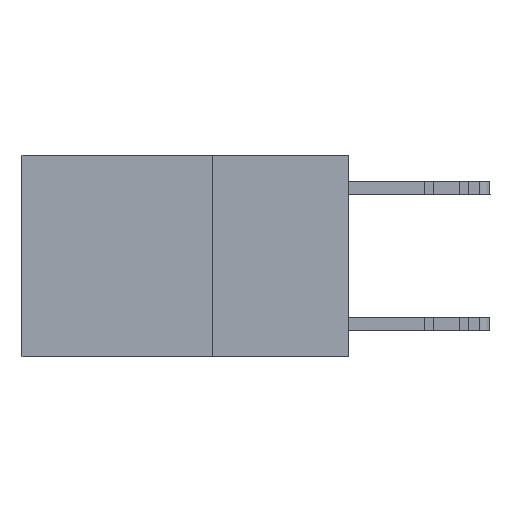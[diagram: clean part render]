
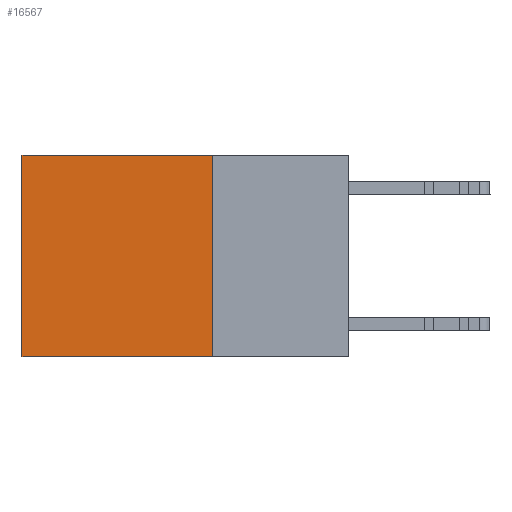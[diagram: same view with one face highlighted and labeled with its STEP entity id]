
A CAD part, left-side view. The second image highlights one B-rep face of the part: STEP entity #16567.
In plain terms, the highlighted planar face has unit normal (-1, 0, 0).
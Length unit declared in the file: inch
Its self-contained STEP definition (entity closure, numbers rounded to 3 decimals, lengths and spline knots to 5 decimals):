
#585 = ORIENTED_EDGE ( 'NONE', *, *, #17631, .T. ) ;
#606 = CARTESIAN_POINT ( 'NONE',  ( 0.2625, 0.25, 0. ) ) ;
#1073 = VECTOR ( 'NONE', #25518, 39.37008 ) ;
#1113 = EDGE_CURVE ( 'NONE', #17965, #26983, #7834, .T. ) ;
#1301 = LINE ( 'NONE', #3495, #11251 ) ;
#2492 = LINE ( 'NONE', #8515, #1073 ) ;
#2721 = PLANE ( 'NONE',  #20192 ) ;
#3495 = CARTESIAN_POINT ( 'NONE',  ( 0.2625, 0.25, -0.37 ) ) ;
#3881 = CARTESIAN_POINT ( 'NONE',  ( 0.2625, 0.25, 0. ) ) ;
#4057 = DIRECTION ( 'NONE',  ( 0., 0., -1. ) ) ;
#4924 = DIRECTION ( 'NONE',  ( 0., 0., -1. ) ) ;
#5429 = VECTOR ( 'NONE', #28296, 39.37008 ) ;
#5639 = DIRECTION ( 'NONE',  ( 1., 0., 0. ) ) ;
#6113 = ORIENTED_EDGE ( 'NONE', *, *, #12246, .T. ) ;
#6474 = CARTESIAN_POINT ( 'NONE',  ( 0.2625, 0.6, -0.37 ) ) ;
#7419 = CARTESIAN_POINT ( 'NONE',  ( 0.2625, 0.25, -0.37 ) ) ;
#7834 = LINE ( 'NONE', #22154, #13680 ) ;
#8515 = CARTESIAN_POINT ( 'NONE',  ( 0.2625, 0.25, 0. ) ) ;
#9841 = VERTEX_POINT ( 'NONE', #15784 ) ;
#11021 = VERTEX_POINT ( 'NONE', #6474 ) ;
#11251 = VECTOR ( 'NONE', #17276, 39.37008 ) ;
#12246 = EDGE_CURVE ( 'NONE', #17965, #9841, #2492, .T. ) ;
#13680 = VECTOR ( 'NONE', #4057, 39.37008 ) ;
#14698 = ORIENTED_EDGE ( 'NONE', *, *, #24680, .F. ) ;
#15700 = CARTESIAN_POINT ( 'NONE',  ( 0.2625, 0.6, 0. ) ) ;
#15784 = CARTESIAN_POINT ( 'NONE',  ( 0.2625, 0.6, 0. ) ) ;
#16567 = ADVANCED_FACE ( 'NONE', ( #21481 ), #2721, .F. ) ;
#17276 = DIRECTION ( 'NONE',  ( 0., 1., 0. ) ) ;
#17631 = EDGE_CURVE ( 'NONE', #9841, #11021, #28274, .T. ) ;
#17965 = VERTEX_POINT ( 'NONE', #3881 ) ;
#18042 = EDGE_LOOP ( 'NONE', ( #585, #14698, #19778, #6113 ) ) ;
#19778 = ORIENTED_EDGE ( 'NONE', *, *, #1113, .F. ) ;
#20192 = AXIS2_PLACEMENT_3D ( 'NONE', #606, #5639, #4924 ) ;
#21481 = FACE_OUTER_BOUND ( 'NONE', #18042, .T. ) ;
#22154 = CARTESIAN_POINT ( 'NONE',  ( 0.2625, 0.25, 0. ) ) ;
#24680 = EDGE_CURVE ( 'NONE', #26983, #11021, #1301, .T. ) ;
#25518 = DIRECTION ( 'NONE',  ( 0., 1., 0. ) ) ;
#26983 = VERTEX_POINT ( 'NONE', #7419 ) ;
#28274 = LINE ( 'NONE', #15700, #5429 ) ;
#28296 = DIRECTION ( 'NONE',  ( 0., 0., -1. ) ) ;
